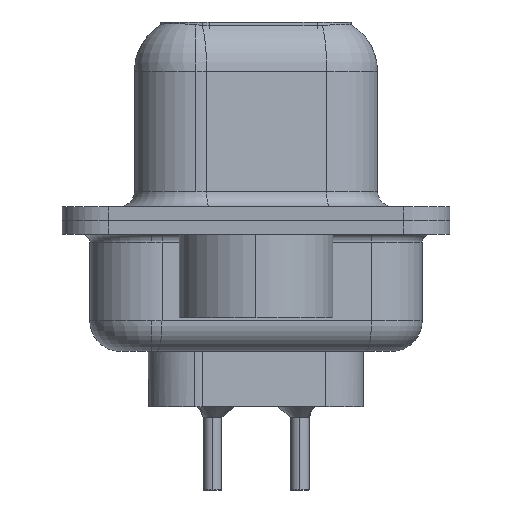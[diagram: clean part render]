
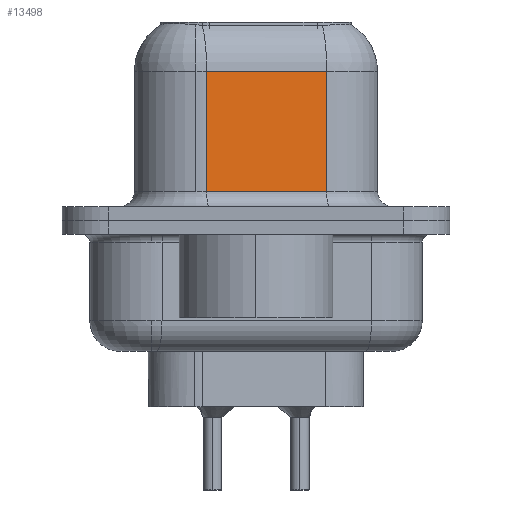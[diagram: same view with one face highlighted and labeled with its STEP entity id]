
A CAD part, left-side view. The second image highlights one B-rep face of the part: STEP entity #13498.
In plain terms, the highlighted planar face has unit normal (-0.985, -0.174, 0).
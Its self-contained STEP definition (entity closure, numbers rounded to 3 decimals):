
#28 = DIRECTION ( 'NONE',  ( 0.174, -0.985, 0. ) ) ;
#109 = CARTESIAN_POINT ( 'NONE',  ( 5.063, -2.297, 0.95 ) ) ;
#516 = EDGE_CURVE ( 'NONE', #4832, #16527, #10449, .T. ) ;
#634 = LINE ( 'NONE', #17808, #17923 ) ;
#687 = EDGE_LOOP ( 'NONE', ( #13660, #14503, #18091, #14805 ) ) ;
#1134 = DIRECTION ( 'NONE',  ( -0.174, 0.985, 0. ) ) ;
#1563 = VECTOR ( 'NONE', #1134, 1000. ) ;
#2459 = CARTESIAN_POINT ( 'NONE',  ( 5.063, -2.297, 6.6 ) ) ;
#2603 = EDGE_CURVE ( 'NONE', #19214, #10770, #18843, .T. ) ;
#4832 = VERTEX_POINT ( 'NONE', #15248 ) ;
#6548 = CARTESIAN_POINT ( 'NONE',  ( 5.063, -2.297, 4.85 ) ) ;
#6965 = CARTESIAN_POINT ( 'NONE',  ( 5.063, -2.297, 6.6 ) ) ;
#7773 = DIRECTION ( 'NONE',  ( 0., 0., -1. ) ) ;
#8566 = PLANE ( 'NONE',  #14704 ) ;
#8623 = DIRECTION ( 'NONE',  ( -0.174, 0.985, 0. ) ) ;
#9182 = DIRECTION ( 'NONE',  ( 0., 0., -1. ) ) ;
#10449 = LINE ( 'NONE', #6548, #1563 ) ;
#10770 = VERTEX_POINT ( 'NONE', #20402 ) ;
#10997 = EDGE_CURVE ( 'NONE', #4832, #10770, #18649, .T. ) ;
#11527 = CARTESIAN_POINT ( 'NONE',  ( 4.375, 1.603, 0.95 ) ) ;
#11714 = FACE_OUTER_BOUND ( 'NONE', #687, .T. ) ;
#13498 = ADVANCED_FACE ( 'NONE', ( #11714 ), #8566, .F. ) ;
#13660 = ORIENTED_EDGE ( 'NONE', *, *, #10997, .F. ) ;
#14155 = VECTOR ( 'NONE', #9182, 1000. ) ;
#14503 = ORIENTED_EDGE ( 'NONE', *, *, #516, .T. ) ;
#14704 = AXIS2_PLACEMENT_3D ( 'NONE', #6965, #18697, #8623 ) ;
#14805 = ORIENTED_EDGE ( 'NONE', *, *, #2603, .T. ) ;
#14873 = VECTOR ( 'NONE', #28, 1000. ) ;
#15248 = CARTESIAN_POINT ( 'NONE',  ( 5.063, -2.297, 4.85 ) ) ;
#16427 = CARTESIAN_POINT ( 'NONE',  ( 4.375, 1.603, 4.85 ) ) ;
#16527 = VERTEX_POINT ( 'NONE', #16427 ) ;
#17808 = CARTESIAN_POINT ( 'NONE',  ( 4.375, 1.603, 6.6 ) ) ;
#17923 = VECTOR ( 'NONE', #7773, 1000. ) ;
#18091 = ORIENTED_EDGE ( 'NONE', *, *, #21577, .T. ) ;
#18649 = LINE ( 'NONE', #2459, #14155 ) ;
#18697 = DIRECTION ( 'NONE',  ( 0.985, 0.174, 0. ) ) ;
#18843 = LINE ( 'NONE', #109, #14873 ) ;
#19214 = VERTEX_POINT ( 'NONE', #11527 ) ;
#20402 = CARTESIAN_POINT ( 'NONE',  ( 5.063, -2.297, 0.95 ) ) ;
#21577 = EDGE_CURVE ( 'NONE', #16527, #19214, #634, .T. ) ;
